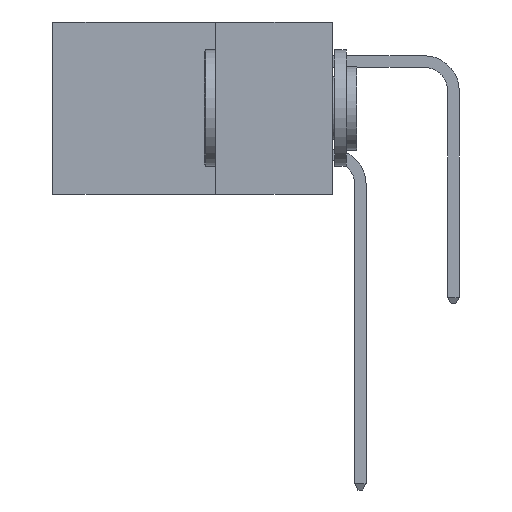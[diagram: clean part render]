
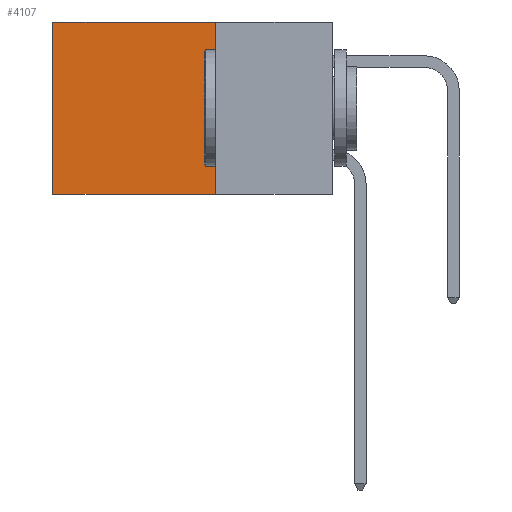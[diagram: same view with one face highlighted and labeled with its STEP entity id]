
A CAD part, left-side view. The second image highlights one B-rep face of the part: STEP entity #4107.
In plain terms, the highlighted planar face has unit normal (-1, 0, 0).
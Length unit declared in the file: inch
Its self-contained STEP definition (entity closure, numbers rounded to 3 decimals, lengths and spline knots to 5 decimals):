
#107 = DIRECTION ( 'NONE',  ( 0., 1., 0. ) ) ;
#306 = DIRECTION ( 'NONE',  ( 0., 0., -1. ) ) ;
#1318 = CARTESIAN_POINT ( 'NONE',  ( 0.2615, 0.25, 0. ) ) ;
#2624 = EDGE_LOOP ( 'NONE', ( #14581, #7572, #23336, #24409 ) ) ;
#4107 = ADVANCED_FACE ( 'NONE', ( #20887 ), #18890, .F. ) ;
#4148 = VERTEX_POINT ( 'NONE', #18141 ) ;
#6352 = CARTESIAN_POINT ( 'NONE',  ( 0.2615, 0.25, -0.37 ) ) ;
#7339 = EDGE_CURVE ( 'NONE', #9239, #4148, #24839, .T. ) ;
#7572 = ORIENTED_EDGE ( 'NONE', *, *, #18210, .F. ) ;
#8156 = EDGE_CURVE ( 'NONE', #4148, #14713, #25421, .T. ) ;
#8512 = CARTESIAN_POINT ( 'NONE',  ( 0.2615, 0.6, -0.37 ) ) ;
#8589 = VECTOR ( 'NONE', #306, 39.37008 ) ;
#8887 = CARTESIAN_POINT ( 'NONE',  ( 0.2615, 0.25, -0.37 ) ) ;
#9064 = VECTOR ( 'NONE', #107, 39.37008 ) ;
#9239 = VERTEX_POINT ( 'NONE', #20620 ) ;
#9486 = VECTOR ( 'NONE', #18610, 39.37008 ) ;
#12165 = EDGE_CURVE ( 'NONE', #9239, #12913, #19775, .T. ) ;
#12888 = CARTESIAN_POINT ( 'NONE',  ( 0.2615, 0.25, -0.37 ) ) ;
#12913 = VERTEX_POINT ( 'NONE', #8887 ) ;
#14581 = ORIENTED_EDGE ( 'NONE', *, *, #8156, .T. ) ;
#14713 = VERTEX_POINT ( 'NONE', #8512 ) ;
#17447 = VECTOR ( 'NONE', #18081, 39.37008 ) ;
#18081 = DIRECTION ( 'NONE',  ( 0., 1., 0. ) ) ;
#18141 = CARTESIAN_POINT ( 'NONE',  ( 0.2615, 0.6, 0. ) ) ;
#18210 = EDGE_CURVE ( 'NONE', #12913, #14713, #25625, .T. ) ;
#18610 = DIRECTION ( 'NONE',  ( 0., 0., -1. ) ) ;
#18823 = DIRECTION ( 'NONE',  ( 0., 0., -1. ) ) ;
#18829 = DIRECTION ( 'NONE',  ( 1., 0., 0. ) ) ;
#18890 = PLANE ( 'NONE',  #19079 ) ;
#19067 = CARTESIAN_POINT ( 'NONE',  ( 0.2615, 0.25, -0.37 ) ) ;
#19079 = AXIS2_PLACEMENT_3D ( 'NONE', #19067, #18829, #18823 ) ;
#19775 = LINE ( 'NONE', #12888, #8589 ) ;
#20620 = CARTESIAN_POINT ( 'NONE',  ( 0.2615, 0.25, 0. ) ) ;
#20777 = CARTESIAN_POINT ( 'NONE',  ( 0.2615, 0.6, -0.37 ) ) ;
#20887 = FACE_OUTER_BOUND ( 'NONE', #2624, .T. ) ;
#23336 = ORIENTED_EDGE ( 'NONE', *, *, #12165, .F. ) ;
#24409 = ORIENTED_EDGE ( 'NONE', *, *, #7339, .T. ) ;
#24839 = LINE ( 'NONE', #1318, #17447 ) ;
#25421 = LINE ( 'NONE', #20777, #9486 ) ;
#25625 = LINE ( 'NONE', #6352, #9064 ) ;
